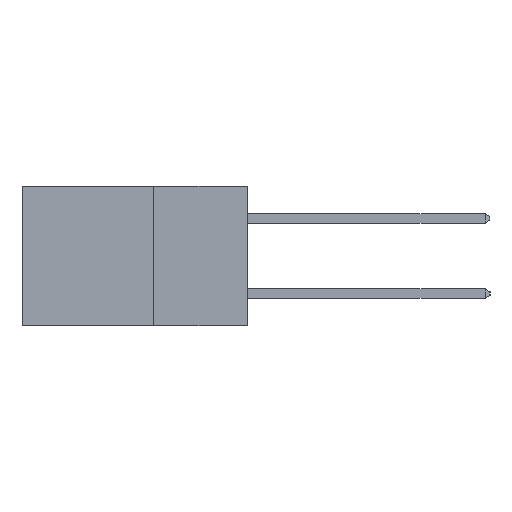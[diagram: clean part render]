
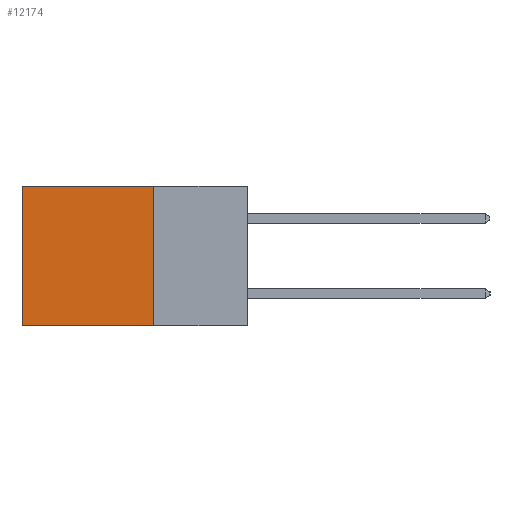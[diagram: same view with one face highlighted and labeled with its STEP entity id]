
A CAD part, left-side view. The second image highlights one B-rep face of the part: STEP entity #12174.
In plain terms, the highlighted planar face has unit normal (-1, 0, 0).
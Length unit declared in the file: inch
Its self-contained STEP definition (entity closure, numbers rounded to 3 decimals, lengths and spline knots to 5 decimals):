
#127 = DIRECTION ( 'NONE',  ( 0., 1., 0. ) ) ;
#636 = CARTESIAN_POINT ( 'NONE',  ( 0.2615, 0.6, -0.37 ) ) ;
#794 = ORIENTED_EDGE ( 'NONE', *, *, #12423, .F. ) ;
#2584 = LINE ( 'NONE', #636, #15241 ) ;
#2811 = ORIENTED_EDGE ( 'NONE', *, *, #11181, .F. ) ;
#2861 = CARTESIAN_POINT ( 'NONE',  ( 0.2615, 0.25, -0.37 ) ) ;
#3697 = EDGE_CURVE ( 'NONE', #12532, #4091, #6656, .T. ) ;
#3895 = VERTEX_POINT ( 'NONE', #2861 ) ;
#4004 = VECTOR ( 'NONE', #127, 39.37008 ) ;
#4091 = VERTEX_POINT ( 'NONE', #9998 ) ;
#4625 = EDGE_CURVE ( 'NONE', #4091, #9663, #2584, .T. ) ;
#5662 = ORIENTED_EDGE ( 'NONE', *, *, #3697, .T. ) ;
#5889 = PLANE ( 'NONE',  #10080 ) ;
#5917 = DIRECTION ( 'NONE',  ( 0., 0., -1. ) ) ;
#6332 = CARTESIAN_POINT ( 'NONE',  ( 0.2615, 0.25, 0. ) ) ;
#6590 = CARTESIAN_POINT ( 'NONE',  ( 0.2615, 0.25, 0. ) ) ;
#6656 = LINE ( 'NONE', #6332, #7047 ) ;
#6867 = LINE ( 'NONE', #7650, #4004 ) ;
#7047 = VECTOR ( 'NONE', #12997, 39.37008 ) ;
#7143 = CARTESIAN_POINT ( 'NONE',  ( 0.2615, 0.25, -0.37 ) ) ;
#7650 = CARTESIAN_POINT ( 'NONE',  ( 0.2615, 0.25, -0.37 ) ) ;
#8070 = LINE ( 'NONE', #12460, #14242 ) ;
#8391 = DIRECTION ( 'NONE',  ( 0., 0., -1. ) ) ;
#8841 = CARTESIAN_POINT ( 'NONE',  ( 0.2615, 0.6, -0.37 ) ) ;
#9663 = VERTEX_POINT ( 'NONE', #8841 ) ;
#9998 = CARTESIAN_POINT ( 'NONE',  ( 0.2615, 0.6, 0. ) ) ;
#10080 = AXIS2_PLACEMENT_3D ( 'NONE', #7143, #15645, #8391 ) ;
#10179 = EDGE_LOOP ( 'NONE', ( #11238, #794, #2811, #5662 ) ) ;
#11181 = EDGE_CURVE ( 'NONE', #12532, #3895, #8070, .T. ) ;
#11238 = ORIENTED_EDGE ( 'NONE', *, *, #4625, .T. ) ;
#12174 = ADVANCED_FACE ( 'NONE', ( #13496 ), #5889, .F. ) ;
#12408 = DIRECTION ( 'NONE',  ( 0., 0., -1. ) ) ;
#12423 = EDGE_CURVE ( 'NONE', #3895, #9663, #6867, .T. ) ;
#12460 = CARTESIAN_POINT ( 'NONE',  ( 0.2615, 0.25, -0.37 ) ) ;
#12532 = VERTEX_POINT ( 'NONE', #6590 ) ;
#12997 = DIRECTION ( 'NONE',  ( 0., 1., 0. ) ) ;
#13496 = FACE_OUTER_BOUND ( 'NONE', #10179, .T. ) ;
#14242 = VECTOR ( 'NONE', #12408, 39.37008 ) ;
#15241 = VECTOR ( 'NONE', #5917, 39.37008 ) ;
#15645 = DIRECTION ( 'NONE',  ( 1., 0., 0. ) ) ;
